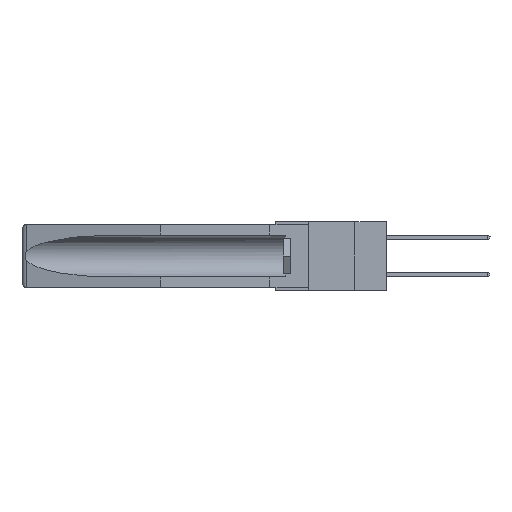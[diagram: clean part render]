
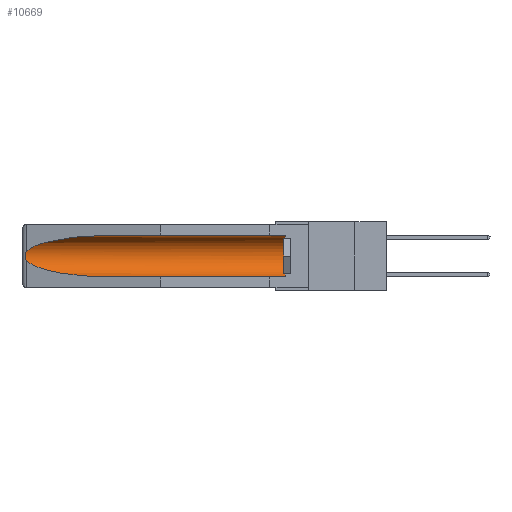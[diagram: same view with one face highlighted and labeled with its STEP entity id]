
A CAD part, left-side view. The second image highlights one B-rep face of the part: STEP entity #10669.
In plain terms, the highlighted cylindrical face has radius 2.857 mm (diameter 5.715 mm), a partial arc.
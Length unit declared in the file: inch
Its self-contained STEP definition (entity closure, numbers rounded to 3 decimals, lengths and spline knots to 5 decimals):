
#3 = CARTESIAN_POINT ( 'NONE',  ( 0.25451, 1.48313, -0.09465 ) ) ;
#261 = DIRECTION ( 'NONE',  ( 0., -1., 0. ) ) ;
#473 = DIRECTION ( 'NONE',  ( 0., 0., 1. ) ) ;
#490 = CARTESIAN_POINT ( 'NONE',  ( 0.26537, 1.52718, -0.14972 ) ) ;
#624 = AXIS2_PLACEMENT_3D ( 'NONE', #9603, #22009, #6681 ) ;
#723 = CARTESIAN_POINT ( 'NONE',  ( 0.2673, 1.5327, -0.16383 ) ) ;
#1030 = CARTESIAN_POINT ( 'NONE',  ( 0.26537, 1.52718, -0.19328 ) ) ;
#1143 = ORIENTED_EDGE ( 'NONE', *, *, #13606, .T. ) ;
#1531 = EDGE_CURVE ( 'NONE', #5338, #9307, #22087, .T. ) ;
#2576 = CARTESIAN_POINT ( 'NONE',  ( 0.2675, 1.53308, -0.16763 ) ) ;
#2652 = EDGE_CURVE ( 'NONE', #13938, #16687, #18485, .T. ) ;
#3778 = CARTESIAN_POINT ( 'NONE',  ( 0.155, 0.126, -0.1715 ) ) ;
#3960 =( BOUNDED_CURVE ( )  B_SPLINE_CURVE ( 3, ( #14270, #12327, #5258, #12403 ),
 .UNSPECIFIED., .F., .T. ) 
 B_SPLINE_CURVE_WITH_KNOTS ( ( 4, 4 ),
 ( 0.1948, 1.5708 ),
 .UNSPECIFIED. ) 
 CURVE ( )  GEOMETRIC_REPRESENTATION_ITEM ( )  RATIONAL_B_SPLINE_CURVE ( ( 1., 0.848, 0.848, 1. ) ) 
 REPRESENTATION_ITEM ( '' )  );
#4540 = CARTESIAN_POINT ( 'NONE',  ( 0.26597, 1.5296, -0.19026 ) ) ;
#4993 = CIRCLE ( 'NONE', #20933, 0.1125 ) ;
#5258 = CARTESIAN_POINT ( 'NONE',  ( 0.21114, 1.30732, -0.284 ) ) ;
#5338 = VERTEX_POINT ( 'NONE', #17767 ) ;
#6195 = CARTESIAN_POINT ( 'NONE',  ( 0.2675, 1.53308, -0.17534 ) ) ;
#6681 = DIRECTION ( 'NONE',  ( 0., 0., 1. ) ) ;
#6683 = DIRECTION ( 'NONE',  ( 0., 1., 0. ) ) ;
#6697 = EDGE_LOOP ( 'NONE', ( #13820, #15416, #1143, #13776, #19554, #20581 ) ) ;
#8337 = CARTESIAN_POINT ( 'NONE',  ( 0.26537, 1.52718, -0.14972 ) ) ;
#8418 = VERTEX_POINT ( 'NONE', #18732 ) ;
#8632 = CARTESIAN_POINT ( 'NONE',  ( 0.155, -0.30754, -0.284 ) ) ;
#9307 = VERTEX_POINT ( 'NONE', #18535 ) ;
#9474 = LINE ( 'NONE', #14384, #20585 ) ;
#9478 = DIRECTION ( 'NONE',  ( 0., 1., 0. ) ) ;
#9603 = CARTESIAN_POINT ( 'NONE',  ( 0.155, -0.30754, -0.1715 ) ) ;
#9636 = CARTESIAN_POINT ( 'NONE',  ( 0.2673, 1.53269, -0.17917 ) ) ;
#9861 = CARTESIAN_POINT ( 'NONE',  ( 0.26655, 1.53094, -0.18657 ) ) ;
#10669 = ADVANCED_FACE ( 'NONE', ( #20929 ), #15125, .F. ) ;
#11159 = CARTESIAN_POINT ( 'NONE',  ( 0.155, 1.07973, -0.059 ) ) ;
#12327 = CARTESIAN_POINT ( 'NONE',  ( 0.25451, 1.48313, -0.24835 ) ) ;
#12403 = CARTESIAN_POINT ( 'NONE',  ( 0.155, 1.07973, -0.284 ) ) ;
#13606 = EDGE_CURVE ( 'NONE', #17535, #9307, #3960, .T. ) ;
#13776 = ORIENTED_EDGE ( 'NONE', *, *, #1531, .F. ) ;
#13820 = ORIENTED_EDGE ( 'NONE', *, *, #2652, .T. ) ;
#13938 = VERTEX_POINT ( 'NONE', #11159 ) ;
#14127 = EDGE_CURVE ( 'NONE', #8418, #13938, #9474, .T. ) ;
#14196 = CARTESIAN_POINT ( 'NONE',  ( 0.26537, 1.52718, -0.14972 ) ) ;
#14270 = CARTESIAN_POINT ( 'NONE',  ( 0.26537, 1.52718, -0.19328 ) ) ;
#14384 = CARTESIAN_POINT ( 'NONE',  ( 0.155, -0.30754, -0.059 ) ) ;
#15125 = CYLINDRICAL_SURFACE ( 'NONE', #624, 0.1125 ) ;
#15163 = VECTOR ( 'NONE', #6683, 39.37008 ) ;
#15416 = ORIENTED_EDGE ( 'NONE', *, *, #18428, .T. ) ;
#15776 = CARTESIAN_POINT ( 'NONE',  ( 0.26654, 1.53092, -0.15636 ) ) ;
#16687 = VERTEX_POINT ( 'NONE', #490 ) ;
#17535 = VERTEX_POINT ( 'NONE', #19695 ) ;
#17767 = CARTESIAN_POINT ( 'NONE',  ( 0.155, 0.126, -0.284 ) ) ;
#18428 = EDGE_CURVE ( 'NONE', #16687, #17535, #22815, .T. ) ;
#18485 =( BOUNDED_CURVE ( )  B_SPLINE_CURVE ( 3, ( #19452, #19279, #3, #14196 ),
 .UNSPECIFIED., .F., .T. ) 
 B_SPLINE_CURVE_WITH_KNOTS ( ( 4, 4 ),
 ( 4.71239, 6.08839 ),
 .UNSPECIFIED. ) 
 CURVE ( )  GEOMETRIC_REPRESENTATION_ITEM ( )  RATIONAL_B_SPLINE_CURVE ( ( 1., 0.848, 0.848, 1. ) ) 
 REPRESENTATION_ITEM ( '' )  );
#18535 = CARTESIAN_POINT ( 'NONE',  ( 0.155, 1.07973, -0.284 ) ) ;
#18732 = CARTESIAN_POINT ( 'NONE',  ( 0.155, 0.126, -0.059 ) ) ;
#19279 = CARTESIAN_POINT ( 'NONE',  ( 0.21114, 1.30732, -0.059 ) ) ;
#19452 = CARTESIAN_POINT ( 'NONE',  ( 0.155, 1.07973, -0.059 ) ) ;
#19554 = ORIENTED_EDGE ( 'NONE', *, *, #22248, .T. ) ;
#19695 = CARTESIAN_POINT ( 'NONE',  ( 0.26537, 1.52718, -0.19328 ) ) ;
#20581 = ORIENTED_EDGE ( 'NONE', *, *, #14127, .T. ) ;
#20585 = VECTOR ( 'NONE', #9478, 39.37008 ) ;
#20929 = FACE_OUTER_BOUND ( 'NONE', #6697, .T. ) ;
#20933 = AXIS2_PLACEMENT_3D ( 'NONE', #3778, #261, #473 ) ;
#21035 = CARTESIAN_POINT ( 'NONE',  ( 0.26597, 1.52961, -0.15275 ) ) ;
#22009 = DIRECTION ( 'NONE',  ( 0., 1., 0. ) ) ;
#22087 = LINE ( 'NONE', #8632, #15163 ) ;
#22248 = EDGE_CURVE ( 'NONE', #5338, #8418, #4993, .T. ) ;
#22815 = B_SPLINE_CURVE_WITH_KNOTS ( 'NONE', 3,
 ( #8337, #21035, #15776, #723, #2576, #6195, #9636, #9861, #4540, #1030 ),
 .UNSPECIFIED., .F., .F.,
 ( 4, 2, 2, 2, 4 ),
 ( 0., 0.00029, 0.00058, 0.00087, 0.00117 ),
 .UNSPECIFIED. ) ;
